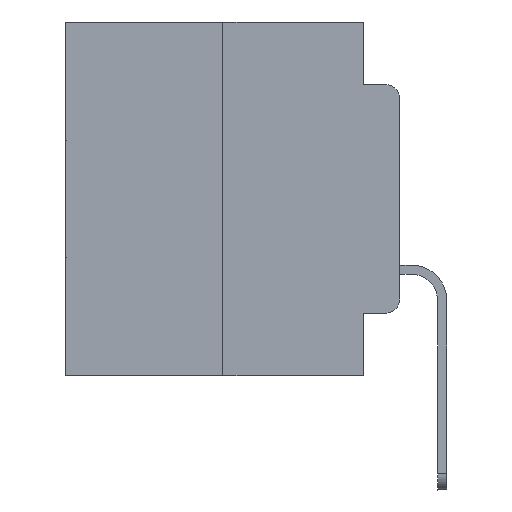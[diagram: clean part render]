
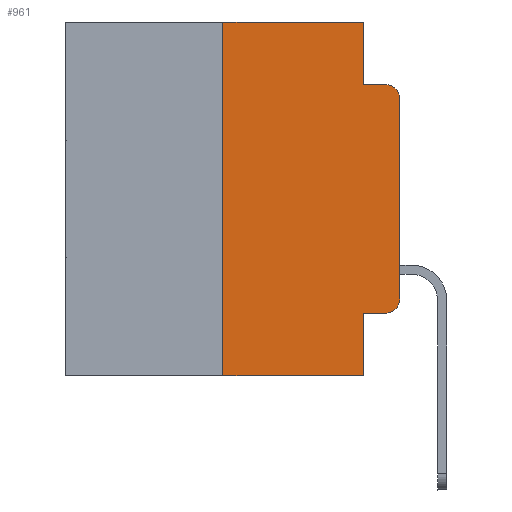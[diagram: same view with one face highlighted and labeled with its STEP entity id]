
A CAD part, left-side view. The second image highlights one B-rep face of the part: STEP entity #961.
In plain terms, the highlighted planar face has unit normal (-1, 0, 0).
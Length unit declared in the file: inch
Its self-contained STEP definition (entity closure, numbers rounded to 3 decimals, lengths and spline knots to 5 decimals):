
#961 = ADVANCED_FACE ( 'NONE', ( #25293 ), #17671, .F. ) ;
#1172 = VERTEX_POINT ( 'NONE', #24582 ) ;
#1183 = DIRECTION ( 'NONE',  ( 0., -1., 0. ) ) ;
#1220 = VERTEX_POINT ( 'NONE', #6334 ) ;
#1319 = CARTESIAN_POINT ( 'NONE',  ( 0., 0.051, -0.4115 ) ) ;
#1476 = EDGE_CURVE ( 'NONE', #4145, #12017, #13348, .T. ) ;
#1755 = DIRECTION ( 'NONE',  ( 0., 0., -1. ) ) ;
#2091 = LINE ( 'NONE', #16730, #24015 ) ;
#2213 = CARTESIAN_POINT ( 'NONE',  ( 0., 0.473, 0. ) ) ;
#2538 = AXIS2_PLACEMENT_3D ( 'NONE', #6983, #4931, #11402 ) ;
#2890 = VERTEX_POINT ( 'NONE', #20249 ) ;
#3100 = ORIENTED_EDGE ( 'NONE', *, *, #1476, .F. ) ;
#3230 = EDGE_CURVE ( 'NONE', #14533, #4107, #20488, .T. ) ;
#3320 = VECTOR ( 'NONE', #5988, 39.37008 ) ;
#3573 = ORIENTED_EDGE ( 'NONE', *, *, #11485, .T. ) ;
#4107 = VERTEX_POINT ( 'NONE', #7776 ) ;
#4119 = VECTOR ( 'NONE', #11746, 39.37008 ) ;
#4145 = VERTEX_POINT ( 'NONE', #17739 ) ;
#4213 = EDGE_CURVE ( 'NONE', #14533, #20661, #25047, .T. ) ;
#4605 = EDGE_CURVE ( 'NONE', #1220, #1172, #26684, .T. ) ;
#4893 = EDGE_CURVE ( 'NONE', #4107, #4145, #10904, .T. ) ;
#4931 = DIRECTION ( 'NONE',  ( -1., 0., 0. ) ) ;
#4986 = DIRECTION ( 'NONE',  ( 1., 0., 0. ) ) ;
#5118 = VECTOR ( 'NONE', #11422, 39.37008 ) ;
#5556 = CARTESIAN_POINT ( 'NONE',  ( 0., 0.051, -0.5 ) ) ;
#5988 = DIRECTION ( 'NONE',  ( 0., 0., 1. ) ) ;
#6173 = DIRECTION ( 'NONE',  ( -1., 0., 0. ) ) ;
#6334 = CARTESIAN_POINT ( 'NONE',  ( 0., 0., -0.3915 ) ) ;
#6883 = ORIENTED_EDGE ( 'NONE', *, *, #16106, .T. ) ;
#6983 = CARTESIAN_POINT ( 'NONE',  ( 0., 0.02, -0.1085 ) ) ;
#7606 = CIRCLE ( 'NONE', #9822, 0.02 ) ;
#7740 = LINE ( 'NONE', #18368, #4119 ) ;
#7745 = CARTESIAN_POINT ( 'NONE',  ( 0., 0., 0. ) ) ;
#7776 = CARTESIAN_POINT ( 'NONE',  ( 0., 0.25, 0. ) ) ;
#8582 = DIRECTION ( 'NONE',  ( 0., 0., -1. ) ) ;
#8836 = DIRECTION ( 'NONE',  ( 0., -1., 0. ) ) ;
#8949 = VECTOR ( 'NONE', #8836, 39.37008 ) ;
#9320 = VECTOR ( 'NONE', #16890, 39.37008 ) ;
#9762 = ORIENTED_EDGE ( 'NONE', *, *, #4213, .T. ) ;
#9822 = AXIS2_PLACEMENT_3D ( 'NONE', #20800, #6173, #1755 ) ;
#10867 = AXIS2_PLACEMENT_3D ( 'NONE', #24457, #4986, #26379 ) ;
#10877 = EDGE_LOOP ( 'NONE', ( #18434, #27037, #11147, #3100, #18808, #21019, #9762, #26105, #6883, #3573 ) ) ;
#10904 = LINE ( 'NONE', #2213, #8949 ) ;
#11147 = ORIENTED_EDGE ( 'NONE', *, *, #26552, .F. ) ;
#11402 = DIRECTION ( 'NONE',  ( 0., 0., -1. ) ) ;
#11422 = DIRECTION ( 'NONE',  ( 0., 0., -1. ) ) ;
#11485 = EDGE_CURVE ( 'NONE', #23276, #1220, #7606, .T. ) ;
#11602 = CARTESIAN_POINT ( 'NONE',  ( 0., 0.051, -0.0885 ) ) ;
#11704 = EDGE_CURVE ( 'NONE', #1172, #2890, #25513, .T. ) ;
#11746 = DIRECTION ( 'NONE',  ( 0., -1., 0. ) ) ;
#12013 = VECTOR ( 'NONE', #16166, 39.37008 ) ;
#12017 = VERTEX_POINT ( 'NONE', #11602 ) ;
#13348 = LINE ( 'NONE', #13615, #5118 ) ;
#13615 = CARTESIAN_POINT ( 'NONE',  ( 0., 0.051, 0. ) ) ;
#13996 = CARTESIAN_POINT ( 'NONE',  ( 0., 0.02, -0.4115 ) ) ;
#14140 = VECTOR ( 'NONE', #1183, 39.37008 ) ;
#14533 = VERTEX_POINT ( 'NONE', #23819 ) ;
#16106 = EDGE_CURVE ( 'NONE', #17494, #23276, #20087, .T. ) ;
#16166 = DIRECTION ( 'NONE',  ( 0., 0., 1. ) ) ;
#16485 = CARTESIAN_POINT ( 'NONE',  ( 0., 0.25, 0. ) ) ;
#16730 = CARTESIAN_POINT ( 'NONE',  ( 0., 0.051, 0. ) ) ;
#16890 = DIRECTION ( 'NONE',  ( 0., -1., 0. ) ) ;
#17494 = VERTEX_POINT ( 'NONE', #1319 ) ;
#17671 = PLANE ( 'NONE',  #10867 ) ;
#17739 = CARTESIAN_POINT ( 'NONE',  ( 0., 0.051, 0. ) ) ;
#18368 = CARTESIAN_POINT ( 'NONE',  ( 0., 0.051, -0.0885 ) ) ;
#18434 = ORIENTED_EDGE ( 'NONE', *, *, #4605, .T. ) ;
#18685 = CARTESIAN_POINT ( 'NONE',  ( 0., 0.473, -0.5 ) ) ;
#18808 = ORIENTED_EDGE ( 'NONE', *, *, #4893, .F. ) ;
#20087 = LINE ( 'NONE', #22556, #14140 ) ;
#20249 = CARTESIAN_POINT ( 'NONE',  ( 0., 0.02, -0.0885 ) ) ;
#20488 = LINE ( 'NONE', #16485, #3320 ) ;
#20661 = VERTEX_POINT ( 'NONE', #5556 ) ;
#20800 = CARTESIAN_POINT ( 'NONE',  ( 0., 0.02, -0.3915 ) ) ;
#21019 = ORIENTED_EDGE ( 'NONE', *, *, #3230, .F. ) ;
#22556 = CARTESIAN_POINT ( 'NONE',  ( 0., 0.051, -0.4115 ) ) ;
#23276 = VERTEX_POINT ( 'NONE', #13996 ) ;
#23819 = CARTESIAN_POINT ( 'NONE',  ( 0., 0.25, -0.5 ) ) ;
#24015 = VECTOR ( 'NONE', #8582, 39.37008 ) ;
#24457 = CARTESIAN_POINT ( 'NONE',  ( 0., 0.473, 0. ) ) ;
#24582 = CARTESIAN_POINT ( 'NONE',  ( 0., 0., -0.1085 ) ) ;
#24909 = EDGE_CURVE ( 'NONE', #17494, #20661, #2091, .T. ) ;
#25047 = LINE ( 'NONE', #18685, #9320 ) ;
#25293 = FACE_OUTER_BOUND ( 'NONE', #10877, .T. ) ;
#25513 = CIRCLE ( 'NONE', #2538, 0.02 ) ;
#26105 = ORIENTED_EDGE ( 'NONE', *, *, #24909, .F. ) ;
#26379 = DIRECTION ( 'NONE',  ( 0., 0., -1. ) ) ;
#26552 = EDGE_CURVE ( 'NONE', #12017, #2890, #7740, .T. ) ;
#26684 = LINE ( 'NONE', #7745, #12013 ) ;
#27037 = ORIENTED_EDGE ( 'NONE', *, *, #11704, .T. ) ;
